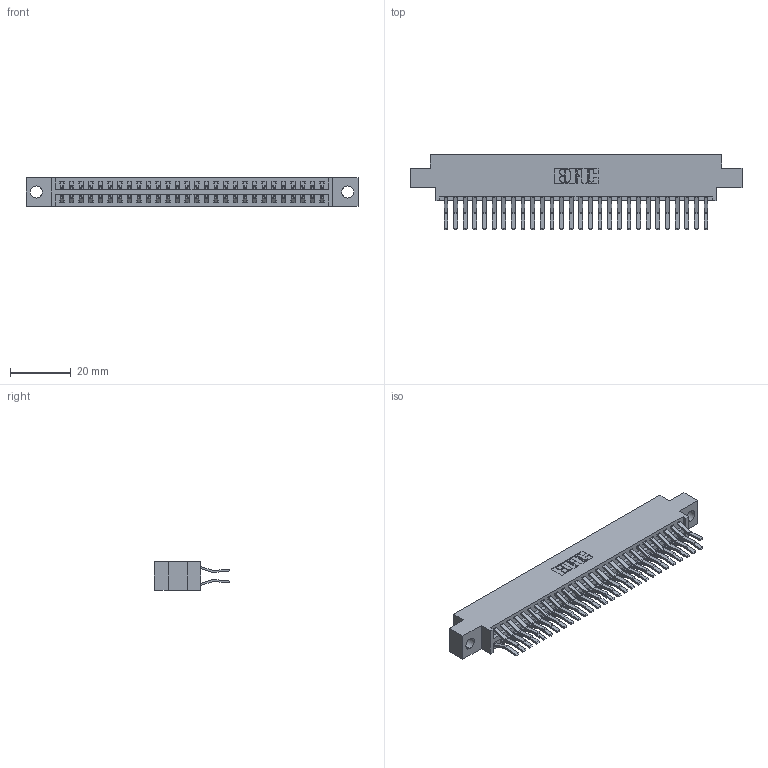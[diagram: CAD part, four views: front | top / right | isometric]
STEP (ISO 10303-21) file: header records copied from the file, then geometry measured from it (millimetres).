
FILE_DESCRIPTION (( 'STEP AP203' ), '1' );
FILE_NAME ('346-056-560-804.STEP', '2018-08-28T03:30:10', ( '' ), ( '' ), 'SwSTEP 2.0', 'SolidWorks 2016', '' );
FILE_SCHEMA (( 'CONFIG_CONTROL_DESIGN' ));
Length unit declared in the file: inch
Products named in the file (3): 345-292-001_560 Tail; 346-056-560-804; 346 Part_0.170 Offset - 0.156 Dia-TH
Assembly tree (57 placements, depth 2):
  346-056-560-804
    346 Part_0.170 Offset - 0.156 Dia-TH
    345-292-001_560 Tail  x56
Bounding box: 109.47 x 24.78 x 9.4 mm (x, y, z)
Volume: 10690.9 mm3; surface area: 15447.6 mm2
Topology: 57 solids, 57 shells, 3150 faces, 9357 edges, 6162 vertices
Faces by surface type: plane 2040, cylinder 1110
Entity records: 20381 total; most frequent: CARTESIAN_POINT 3380, ORIENTED_EDGE 3314, DIRECTION 3033, EDGE_CURVE 1657, LINE 1409, VECTOR 1409, VERTEX_POINT 1102, AXIS2_PLACEMENT_3D 812
